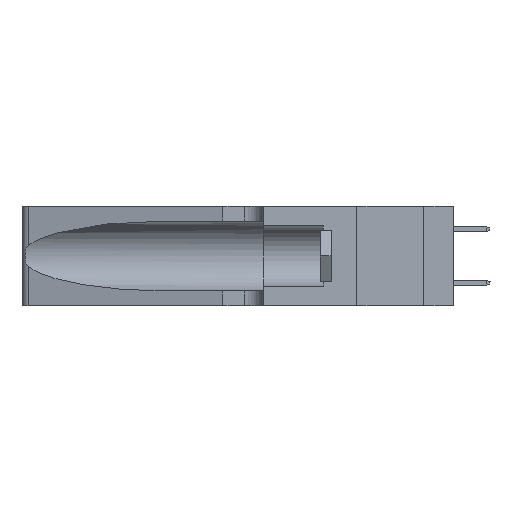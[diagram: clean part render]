
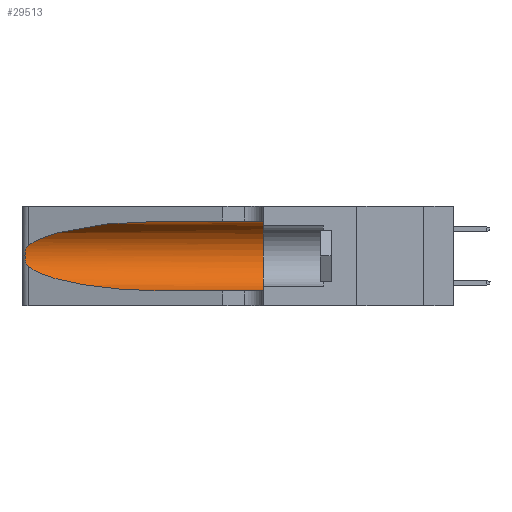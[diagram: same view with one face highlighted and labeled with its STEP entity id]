
A CAD part, left-side view. The second image highlights one B-rep face of the part: STEP entity #29513.
In plain terms, the highlighted cylindrical face has radius 3.308 mm (diameter 6.617 mm), a partial arc.
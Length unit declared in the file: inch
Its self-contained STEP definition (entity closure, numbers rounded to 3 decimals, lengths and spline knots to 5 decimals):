
#1705 = CARTESIAN_POINT ( 'NONE',  ( 0.25487, 1.22718, 0.22369 ) ) ;
#1917 = CARTESIAN_POINT ( 'NONE',  ( 0.26018, 1.23835, 0.19895 ) ) ;
#2228 = B_SPLINE_CURVE_WITH_KNOTS ( 'NONE', 3,
 ( #5491, #16988, #23743, #5300, #5695, #1917, #23352, #2309, #14408, #35675, #35472, #36060, #8271, #32499 ),
 .UNSPECIFIED., .F., .F.,
 ( 4, 2, 2, 2, 2, 2, 4 ),
 ( 0., 0.00027, 0.00053, 0.00107, 0.0016, 0.00187, 0.00214 ),
 .UNSPECIFIED. ) ;
#2309 = CARTESIAN_POINT ( 'NONE',  ( 0.26075, 1.23896, 0.178 ) ) ;
#4015 = CARTESIAN_POINT ( 'NONE',  ( 0.2373, 1.15595, 0.08982 ) ) ;
#4108 = ORIENTED_EDGE ( 'NONE', *, *, #27807, .F. ) ;
#4546 = VERTEX_POINT ( 'NONE', #38794 ) ;
#4681 = VERTEX_POINT ( 'NONE', #27442 ) ;
#5300 = CARTESIAN_POINT ( 'NONE',  ( 0.25787, 1.23484, 0.2124 ) ) ;
#5491 = CARTESIAN_POINT ( 'NONE',  ( 0.25487, 1.22718, 0.22369 ) ) ;
#5695 = CARTESIAN_POINT ( 'NONE',  ( 0.25854, 1.2359, 0.20912 ) ) ;
#6989 = CARTESIAN_POINT ( 'NONE',  ( 0.1305, 0.72297, 0.05475 ) ) ;
#7741 = DIRECTION ( 'NONE',  ( 0., -1., 0. ) ) ;
#7933 = CARTESIAN_POINT ( 'NONE',  ( 0.1305, 1.61858, 0.05475 ) ) ;
#8271 = CARTESIAN_POINT ( 'NONE',  ( 0.25555, 1.22993, 0.14849 ) ) ;
#9076 = VECTOR ( 'NONE', #7741, 39.37008 ) ;
#9226 =( BOUNDED_CURVE ( )  B_SPLINE_CURVE ( 3, ( #19068, #4015, #21859, #6989 ),
 .UNSPECIFIED., .F., .T. ) 
 B_SPLINE_CURVE_WITH_KNOTS ( ( 4, 4 ),
 ( 3.44316, 4.71239 ),
 .UNSPECIFIED. ) 
 CURVE ( )  GEOMETRIC_REPRESENTATION_ITEM ( )  RATIONAL_B_SPLINE_CURVE ( ( 1., 0.87, 0.87, 1. ) ) 
 REPRESENTATION_ITEM ( '' )  );
#9478 = DIRECTION ( 'NONE',  ( 0., 1., 0. ) ) ;
#10022 = CARTESIAN_POINT ( 'NONE',  ( 0.1305, 0.35, 0.31525 ) ) ;
#10448 = EDGE_CURVE ( 'NONE', #21693, #27962, #9226, .T. ) ;
#11823 = FACE_OUTER_BOUND ( 'NONE', #28580, .T. ) ;
#14408 = CARTESIAN_POINT ( 'NONE',  ( 0.26017, 1.23833, 0.17102 ) ) ;
#15116 = EDGE_CURVE ( 'NONE', #27962, #33047, #19810, .T. ) ;
#16199 = CARTESIAN_POINT ( 'NONE',  ( 0.1305, 0.72297, 0.31525 ) ) ;
#16988 = CARTESIAN_POINT ( 'NONE',  ( 0.25555, 1.22994, 0.2215 ) ) ;
#17488 = EDGE_CURVE ( 'NONE', #4546, #31072, #22034, .T. ) ;
#18138 = AXIS2_PLACEMENT_3D ( 'NONE', #30106, #23948, #26136 ) ;
#18594 = CARTESIAN_POINT ( 'NONE',  ( 0.1305, 0.35, 0.185 ) ) ;
#19068 = CARTESIAN_POINT ( 'NONE',  ( 0.25487, 1.22718, 0.14631 ) ) ;
#19810 = LINE ( 'NONE', #7933, #9076 ) ;
#21693 = VERTEX_POINT ( 'NONE', #27370 ) ;
#21859 = CARTESIAN_POINT ( 'NONE',  ( 0.18966, 0.96281, 0.05475 ) ) ;
#22034 = LINE ( 'NONE', #33977, #26243 ) ;
#23043 = ORIENTED_EDGE ( 'NONE', *, *, #15116, .T. ) ;
#23352 = CARTESIAN_POINT ( 'NONE',  ( 0.26075, 1.23896, 0.19203 ) ) ;
#23743 = CARTESIAN_POINT ( 'NONE',  ( 0.25639, 1.23184, 0.21858 ) ) ;
#23911 = EDGE_CURVE ( 'NONE', #4681, #21693, #2228, .T. ) ;
#23948 = DIRECTION ( 'NONE',  ( 0., -1., 0. ) ) ;
#24025 = CARTESIAN_POINT ( 'NONE',  ( 0.1305, 0.35, 0.05475 ) ) ;
#24646 = ORIENTED_EDGE ( 'NONE', *, *, #17488, .F. ) ;
#25642 = CIRCLE ( 'NONE', #35808, 0.13025 ) ;
#25935 = CARTESIAN_POINT ( 'NONE',  ( 0.1305, 0.72297, 0.05475 ) ) ;
#26136 = DIRECTION ( 'NONE',  ( 0., 0., -1. ) ) ;
#26243 = VECTOR ( 'NONE', #27596, 39.37008 ) ;
#26723 = CYLINDRICAL_SURFACE ( 'NONE', #18138, 0.13025 ) ;
#27370 = CARTESIAN_POINT ( 'NONE',  ( 0.25487, 1.22718, 0.14631 ) ) ;
#27442 = CARTESIAN_POINT ( 'NONE',  ( 0.25487, 1.22718, 0.22369 ) ) ;
#27596 = DIRECTION ( 'NONE',  ( 0., -1., 0. ) ) ;
#27807 = EDGE_CURVE ( 'NONE', #31072, #33047, #25642, .T. ) ;
#27962 = VERTEX_POINT ( 'NONE', #25935 ) ;
#28190 = ORIENTED_EDGE ( 'NONE', *, *, #39079, .T. ) ;
#28580 = EDGE_LOOP ( 'NONE', ( #28190, #38074, #32213, #23043, #4108, #24646 ) ) ;
#28711 = CARTESIAN_POINT ( 'NONE',  ( 0.2373, 1.15595, 0.28018 ) ) ;
#29513 = ADVANCED_FACE ( 'NONE', ( #11823 ), #26723, .F. ) ;
#30106 = CARTESIAN_POINT ( 'NONE',  ( 0.1305, 1.61858, 0.185 ) ) ;
#30917 = DIRECTION ( 'NONE',  ( 0., 0., 1. ) ) ;
#31072 = VERTEX_POINT ( 'NONE', #10022 ) ;
#32213 = ORIENTED_EDGE ( 'NONE', *, *, #10448, .T. ) ;
#32499 = CARTESIAN_POINT ( 'NONE',  ( 0.25487, 1.22718, 0.14631 ) ) ;
#33047 = VERTEX_POINT ( 'NONE', #24025 ) ;
#33977 = CARTESIAN_POINT ( 'NONE',  ( 0.1305, 1.61858, 0.31525 ) ) ;
#34680 = CARTESIAN_POINT ( 'NONE',  ( 0.18966, 0.96281, 0.31525 ) ) ;
#35472 = CARTESIAN_POINT ( 'NONE',  ( 0.25789, 1.23486, 0.15765 ) ) ;
#35675 = CARTESIAN_POINT ( 'NONE',  ( 0.25856, 1.23593, 0.16098 ) ) ;
#35808 = AXIS2_PLACEMENT_3D ( 'NONE', #18594, #9478, #30917 ) ;
#36060 = CARTESIAN_POINT ( 'NONE',  ( 0.25639, 1.23186, 0.15144 ) ) ;
#37646 =( BOUNDED_CURVE ( )  B_SPLINE_CURVE ( 3, ( #16199, #34680, #28711, #1705 ),
 .UNSPECIFIED., .F., .T. ) 
 B_SPLINE_CURVE_WITH_KNOTS ( ( 4, 4 ),
 ( 1.5708, 2.84003 ),
 .UNSPECIFIED. ) 
 CURVE ( )  GEOMETRIC_REPRESENTATION_ITEM ( )  RATIONAL_B_SPLINE_CURVE ( ( 1., 0.87, 0.87, 1. ) ) 
 REPRESENTATION_ITEM ( '' )  );
#38074 = ORIENTED_EDGE ( 'NONE', *, *, #23911, .T. ) ;
#38794 = CARTESIAN_POINT ( 'NONE',  ( 0.1305, 0.72297, 0.31525 ) ) ;
#39079 = EDGE_CURVE ( 'NONE', #4546, #4681, #37646, .T. ) ;
